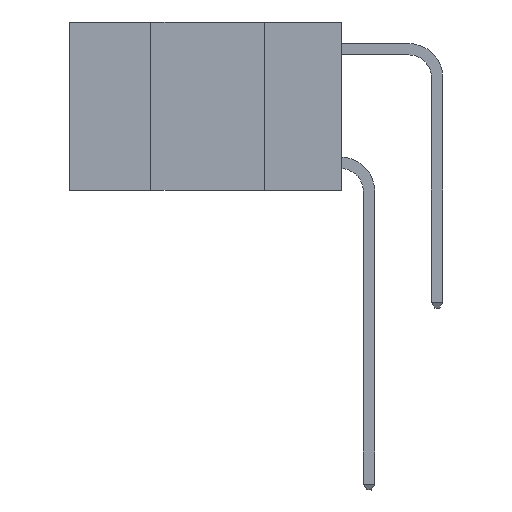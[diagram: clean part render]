
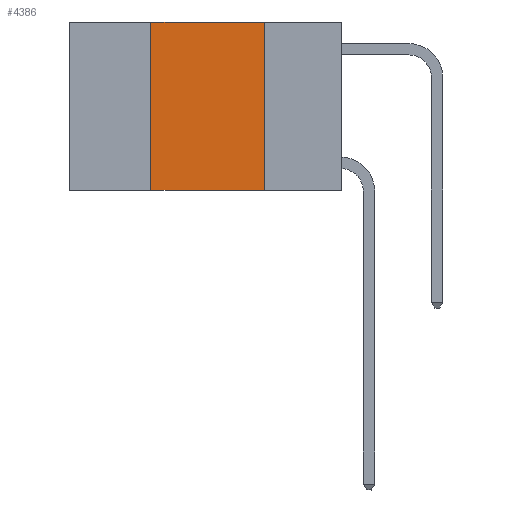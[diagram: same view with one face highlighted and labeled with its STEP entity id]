
A CAD part, left-side view. The second image highlights one B-rep face of the part: STEP entity #4386.
In plain terms, the highlighted planar face has unit normal (-1, 0, 0).
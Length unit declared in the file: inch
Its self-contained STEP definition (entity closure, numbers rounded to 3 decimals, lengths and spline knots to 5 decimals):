
#339 = EDGE_LOOP ( 'NONE', ( #3005, #12213, #12494, #10310 ) ) ;
#477 = CARTESIAN_POINT ( 'NONE',  ( 0., 0.6, 0. ) ) ;
#494 = LINE ( 'NONE', #8893, #6242 ) ;
#585 = LINE ( 'NONE', #6083, #10788 ) ;
#1521 = CARTESIAN_POINT ( 'NONE',  ( 0., 0.17, -0.37 ) ) ;
#2012 = EDGE_CURVE ( 'NONE', #7825, #5339, #494, .T. ) ;
#2484 = CARTESIAN_POINT ( 'NONE',  ( 0., 0.17, 0. ) ) ;
#2601 = DIRECTION ( 'NONE',  ( 1., 0., 0. ) ) ;
#2843 = VECTOR ( 'NONE', #11604, 39.37008 ) ;
#3005 = ORIENTED_EDGE ( 'NONE', *, *, #9743, .F. ) ;
#3391 = DIRECTION ( 'NONE',  ( 0., 0., 1. ) ) ;
#4386 = ADVANCED_FACE ( 'NONE', ( #7061 ), #8831, .F. ) ;
#4989 = CARTESIAN_POINT ( 'NONE',  ( 0., 0.42, -0.37 ) ) ;
#5273 = DIRECTION ( 'NONE',  ( 0., -1., 0. ) ) ;
#5339 = VERTEX_POINT ( 'NONE', #7565 ) ;
#5804 = LINE ( 'NONE', #2484, #2843 ) ;
#5990 = CARTESIAN_POINT ( 'NONE',  ( 0., 0.42, 0. ) ) ;
#6083 = CARTESIAN_POINT ( 'NONE',  ( 0., 0.6, -0.37 ) ) ;
#6242 = VECTOR ( 'NONE', #5273, 39.37008 ) ;
#7061 = FACE_OUTER_BOUND ( 'NONE', #339, .T. ) ;
#7234 = VECTOR ( 'NONE', #3391, 39.37008 ) ;
#7565 = CARTESIAN_POINT ( 'NONE',  ( 0., 0.17, 0. ) ) ;
#7825 = VERTEX_POINT ( 'NONE', #5990 ) ;
#7920 = EDGE_CURVE ( 'NONE', #11071, #12929, #585, .T. ) ;
#8496 = EDGE_CURVE ( 'NONE', #11071, #7825, #10339, .T. ) ;
#8520 = CARTESIAN_POINT ( 'NONE',  ( 0., 0.42, 0. ) ) ;
#8831 = PLANE ( 'NONE',  #12315 ) ;
#8893 = CARTESIAN_POINT ( 'NONE',  ( 0., 0.6, 0. ) ) ;
#9743 = EDGE_CURVE ( 'NONE', #5339, #12929, #5804, .T. ) ;
#9774 = DIRECTION ( 'NONE',  ( 0., 0., -1. ) ) ;
#10310 = ORIENTED_EDGE ( 'NONE', *, *, #7920, .T. ) ;
#10339 = LINE ( 'NONE', #8520, #7234 ) ;
#10788 = VECTOR ( 'NONE', #12732, 39.37008 ) ;
#11071 = VERTEX_POINT ( 'NONE', #4989 ) ;
#11604 = DIRECTION ( 'NONE',  ( 0., 0., -1. ) ) ;
#12213 = ORIENTED_EDGE ( 'NONE', *, *, #2012, .F. ) ;
#12315 = AXIS2_PLACEMENT_3D ( 'NONE', #477, #2601, #9774 ) ;
#12494 = ORIENTED_EDGE ( 'NONE', *, *, #8496, .F. ) ;
#12732 = DIRECTION ( 'NONE',  ( 0., -1., 0. ) ) ;
#12929 = VERTEX_POINT ( 'NONE', #1521 ) ;
